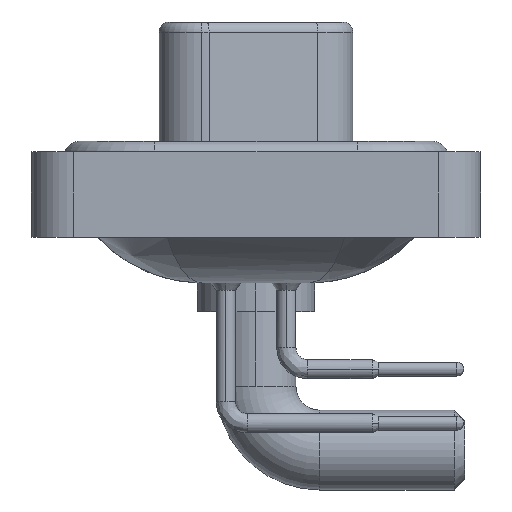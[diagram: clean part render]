
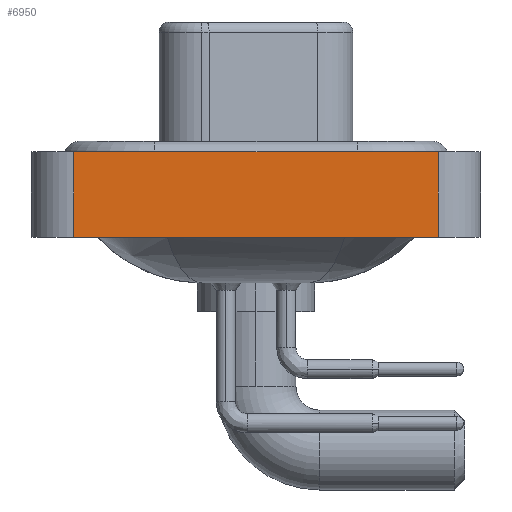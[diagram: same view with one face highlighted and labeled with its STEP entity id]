
A CAD part, left-side view. The second image highlights one B-rep face of the part: STEP entity #6950.
In plain terms, the highlighted planar face has unit normal (-1, 0, 0).
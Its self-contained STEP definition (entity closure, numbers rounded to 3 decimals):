
#77 = CARTESIAN_POINT ( 'NONE',  ( -7.3, 8.55, 0.4 ) ) ;
#402 = ORIENTED_EDGE ( 'NONE', *, *, #25396, .F. ) ;
#1999 = VECTOR ( 'NONE', #5508, 1000. ) ;
#2268 = VERTEX_POINT ( 'NONE', #24208 ) ;
#3236 = EDGE_CURVE ( 'NONE', #2268, #20672, #25411, .T. ) ;
#3921 = LINE ( 'NONE', #7601, #1999 ) ;
#4805 = ORIENTED_EDGE ( 'NONE', *, *, #3236, .T. ) ;
#4876 = CARTESIAN_POINT ( 'NONE',  ( -7.3, -8.55, -3.6 ) ) ;
#5508 = DIRECTION ( 'NONE',  ( 0., 0., 1. ) ) ;
#6337 = EDGE_LOOP ( 'NONE', ( #11441, #402, #16188, #4805 ) ) ;
#6950 = ADVANCED_FACE ( 'NONE', ( #25737 ), #9886, .T. ) ;
#7601 = CARTESIAN_POINT ( 'NONE',  ( -7.3, 8.55, -3.6 ) ) ;
#7782 = CARTESIAN_POINT ( 'NONE',  ( -7.3, -8.55, -3.6 ) ) ;
#8703 = AXIS2_PLACEMENT_3D ( 'NONE', #7782, #15774, #21816 ) ;
#9886 = PLANE ( 'NONE',  #8703 ) ;
#11378 = DIRECTION ( 'NONE',  ( 0., -1., 0. ) ) ;
#11441 = ORIENTED_EDGE ( 'NONE', *, *, #24430, .T. ) ;
#13293 = CARTESIAN_POINT ( 'NONE',  ( -7.3, -8.55, 0.4 ) ) ;
#13732 = EDGE_CURVE ( 'NONE', #2268, #23037, #3921, .T. ) ;
#14632 = LINE ( 'NONE', #24736, #20146 ) ;
#15774 = DIRECTION ( 'NONE',  ( -1., 0., 0. ) ) ;
#16188 = ORIENTED_EDGE ( 'NONE', *, *, #13732, .F. ) ;
#16915 = LINE ( 'NONE', #18902, #19385 ) ;
#16958 = VECTOR ( 'NONE', #11378, 1000. ) ;
#18902 = CARTESIAN_POINT ( 'NONE',  ( -7.3, -8.55, 0.4 ) ) ;
#19045 = VERTEX_POINT ( 'NONE', #13293 ) ;
#19248 = CARTESIAN_POINT ( 'NONE',  ( -7.3, -8.55, -3.6 ) ) ;
#19385 = VECTOR ( 'NONE', #25327, 1000. ) ;
#20146 = VECTOR ( 'NONE', #22152, 1000. ) ;
#20672 = VERTEX_POINT ( 'NONE', #4876 ) ;
#21816 = DIRECTION ( 'NONE',  ( 0., 0., 1. ) ) ;
#22152 = DIRECTION ( 'NONE',  ( 0., 0., 1. ) ) ;
#23037 = VERTEX_POINT ( 'NONE', #77 ) ;
#24208 = CARTESIAN_POINT ( 'NONE',  ( -7.3, 8.55, -3.6 ) ) ;
#24430 = EDGE_CURVE ( 'NONE', #20672, #19045, #14632, .T. ) ;
#24736 = CARTESIAN_POINT ( 'NONE',  ( -7.3, -8.55, -3.6 ) ) ;
#25327 = DIRECTION ( 'NONE',  ( 0., -1., 0. ) ) ;
#25396 = EDGE_CURVE ( 'NONE', #23037, #19045, #16915, .T. ) ;
#25411 = LINE ( 'NONE', #19248, #16958 ) ;
#25737 = FACE_OUTER_BOUND ( 'NONE', #6337, .T. ) ;
